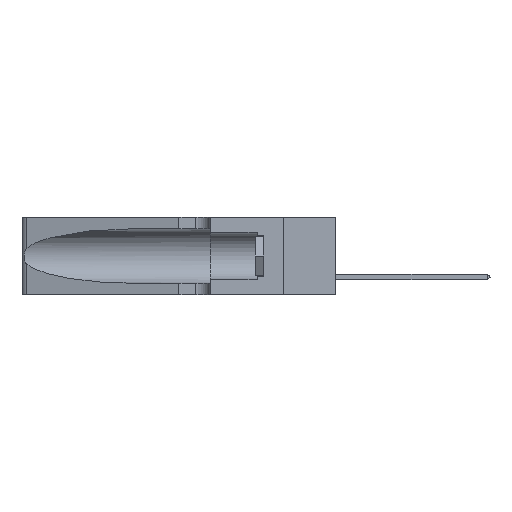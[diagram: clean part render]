
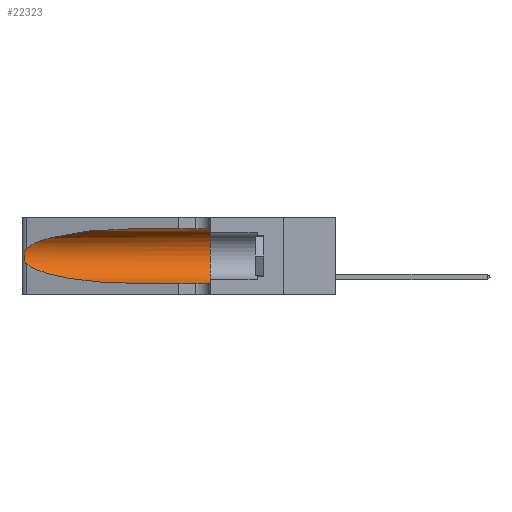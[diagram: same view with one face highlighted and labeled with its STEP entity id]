
A CAD part, left-side view. The second image highlights one B-rep face of the part: STEP entity #22323.
In plain terms, the highlighted cylindrical face has radius 3.308 mm (diameter 6.617 mm), a partial arc.
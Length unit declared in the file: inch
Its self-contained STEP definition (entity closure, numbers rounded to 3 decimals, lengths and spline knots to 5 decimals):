
#426 = ORIENTED_EDGE ( 'NONE', *, *, #15384, .F. ) ;
#1073 = DIRECTION ( 'NONE',  ( 0., 1., 0. ) ) ;
#1305 = CARTESIAN_POINT ( 'NONE',  ( 0.25487, 1.22718, 0.22369 ) ) ;
#1580 = VERTEX_POINT ( 'NONE', #9036 ) ;
#1773 = CARTESIAN_POINT ( 'NONE',  ( 0.18966, 0.96281, 0.05475 ) ) ;
#2220 =( BOUNDED_CURVE ( )  B_SPLINE_CURVE ( 3, ( #8843, #4147, #1773, #11015 ),
 .UNSPECIFIED., .F., .T. ) 
 B_SPLINE_CURVE_WITH_KNOTS ( ( 4, 4 ),
 ( 3.44316, 4.71239 ),
 .UNSPECIFIED. ) 
 CURVE ( )  GEOMETRIC_REPRESENTATION_ITEM ( )  RATIONAL_B_SPLINE_CURVE ( ( 1., 0.87, 0.87, 1. ) ) 
 REPRESENTATION_ITEM ( '' )  );
#3460 = CARTESIAN_POINT ( 'NONE',  ( 0.26075, 1.23896, 0.178 ) ) ;
#3535 = EDGE_CURVE ( 'NONE', #13968, #30046, #26366, .T. ) ;
#4147 = CARTESIAN_POINT ( 'NONE',  ( 0.2373, 1.15595, 0.08982 ) ) ;
#4462 = ORIENTED_EDGE ( 'NONE', *, *, #15866, .T. ) ;
#5500 = ORIENTED_EDGE ( 'NONE', *, *, #24151, .F. ) ;
#5898 = CARTESIAN_POINT ( 'NONE',  ( 0.25854, 1.2359, 0.20912 ) ) ;
#5960 = LINE ( 'NONE', #12563, #29646 ) ;
#5994 = EDGE_CURVE ( 'NONE', #21168, #13968, #2220, .T. ) ;
#6457 = B_SPLINE_CURVE_WITH_KNOTS ( 'NONE', 3,
 ( #1305, #10643, #25045, #27424, #5898, #15581, #17651, #3460, #22440, #8268, #13030, #17847, #24830, #22543 ),
 .UNSPECIFIED., .F., .F.,
 ( 4, 2, 2, 2, 2, 2, 4 ),
 ( 0., 0.00027, 0.00053, 0.00107, 0.0016, 0.00187, 0.00214 ),
 .UNSPECIFIED. ) ;
#7045 = FACE_OUTER_BOUND ( 'NONE', #24908, .T. ) ;
#8268 = CARTESIAN_POINT ( 'NONE',  ( 0.25856, 1.23593, 0.16098 ) ) ;
#8382 = ORIENTED_EDGE ( 'NONE', *, *, #21116, .T. ) ;
#8843 = CARTESIAN_POINT ( 'NONE',  ( 0.25487, 1.22718, 0.14631 ) ) ;
#9036 = CARTESIAN_POINT ( 'NONE',  ( 0.1305, 0.72297, 0.31525 ) ) ;
#9264 = ORIENTED_EDGE ( 'NONE', *, *, #5994, .T. ) ;
#10340 = CARTESIAN_POINT ( 'NONE',  ( 0.1305, 1.61858, 0.185 ) ) ;
#10548 = DIRECTION ( 'NONE',  ( 0., 0., -1. ) ) ;
#10643 = CARTESIAN_POINT ( 'NONE',  ( 0.25555, 1.22994, 0.2215 ) ) ;
#10761 = DIRECTION ( 'NONE',  ( 0., -1., 0. ) ) ;
#10962 = CARTESIAN_POINT ( 'NONE',  ( 0.25487, 1.22718, 0.14631 ) ) ;
#11015 = CARTESIAN_POINT ( 'NONE',  ( 0.1305, 0.72297, 0.05475 ) ) ;
#12563 = CARTESIAN_POINT ( 'NONE',  ( 0.1305, 1.61858, 0.31525 ) ) ;
#13030 = CARTESIAN_POINT ( 'NONE',  ( 0.25789, 1.23486, 0.15765 ) ) ;
#13726 = CARTESIAN_POINT ( 'NONE',  ( 0.18966, 0.96281, 0.31525 ) ) ;
#13968 = VERTEX_POINT ( 'NONE', #14469 ) ;
#14469 = CARTESIAN_POINT ( 'NONE',  ( 0.1305, 0.72297, 0.05475 ) ) ;
#14495 = VECTOR ( 'NONE', #24199, 39.37008 ) ;
#14793 = CYLINDRICAL_SURFACE ( 'NONE', #16896, 0.13025 ) ;
#15261 = CARTESIAN_POINT ( 'NONE',  ( 0.1305, 0.35, 0.185 ) ) ;
#15384 = EDGE_CURVE ( 'NONE', #1580, #29355, #5960, .T. ) ;
#15581 = CARTESIAN_POINT ( 'NONE',  ( 0.26018, 1.23835, 0.19895 ) ) ;
#15806 = AXIS2_PLACEMENT_3D ( 'NONE', #15261, #1073, #19334 ) ;
#15866 = EDGE_CURVE ( 'NONE', #1580, #20215, #21050, .T. ) ;
#16100 = CARTESIAN_POINT ( 'NONE',  ( 0.2373, 1.15595, 0.28018 ) ) ;
#16394 = CARTESIAN_POINT ( 'NONE',  ( 0.1305, 0.72297, 0.31525 ) ) ;
#16896 = AXIS2_PLACEMENT_3D ( 'NONE', #10340, #10761, #10548 ) ;
#17651 = CARTESIAN_POINT ( 'NONE',  ( 0.26075, 1.23896, 0.19203 ) ) ;
#17847 = CARTESIAN_POINT ( 'NONE',  ( 0.25639, 1.23186, 0.15144 ) ) ;
#18046 = ORIENTED_EDGE ( 'NONE', *, *, #3535, .T. ) ;
#18467 = CARTESIAN_POINT ( 'NONE',  ( 0.25487, 1.22718, 0.22369 ) ) ;
#19334 = DIRECTION ( 'NONE',  ( 0., 0., 1. ) ) ;
#19395 = CARTESIAN_POINT ( 'NONE',  ( 0.1305, 1.61858, 0.05475 ) ) ;
#19982 = DIRECTION ( 'NONE',  ( 0., -1., 0. ) ) ;
#20215 = VERTEX_POINT ( 'NONE', #18467 ) ;
#20618 = CIRCLE ( 'NONE', #15806, 0.13025 ) ;
#20868 = CARTESIAN_POINT ( 'NONE',  ( 0.25487, 1.22718, 0.22369 ) ) ;
#21050 =( BOUNDED_CURVE ( )  B_SPLINE_CURVE ( 3, ( #16394, #13726, #16100, #20868 ),
 .UNSPECIFIED., .F., .F. ) 
 B_SPLINE_CURVE_WITH_KNOTS ( ( 4, 4 ),
 ( 1.5708, 2.84003 ),
 .UNSPECIFIED. ) 
 CURVE ( )  GEOMETRIC_REPRESENTATION_ITEM ( )  RATIONAL_B_SPLINE_CURVE ( ( 1., 0.87, 0.87, 1. ) ) 
 REPRESENTATION_ITEM ( '' )  );
#21116 = EDGE_CURVE ( 'NONE', #20215, #21168, #6457, .T. ) ;
#21168 = VERTEX_POINT ( 'NONE', #10962 ) ;
#22323 = ADVANCED_FACE ( 'NONE', ( #7045 ), #14793, .F. ) ;
#22440 = CARTESIAN_POINT ( 'NONE',  ( 0.26017, 1.23833, 0.17102 ) ) ;
#22543 = CARTESIAN_POINT ( 'NONE',  ( 0.25487, 1.22718, 0.14631 ) ) ;
#24151 = EDGE_CURVE ( 'NONE', #29355, #30046, #20618, .T. ) ;
#24199 = DIRECTION ( 'NONE',  ( 0., -1., 0. ) ) ;
#24830 = CARTESIAN_POINT ( 'NONE',  ( 0.25555, 1.22993, 0.14849 ) ) ;
#24908 = EDGE_LOOP ( 'NONE', ( #4462, #8382, #9264, #18046, #5500, #426 ) ) ;
#25045 = CARTESIAN_POINT ( 'NONE',  ( 0.25639, 1.23184, 0.21858 ) ) ;
#26366 = LINE ( 'NONE', #19395, #14495 ) ;
#27424 = CARTESIAN_POINT ( 'NONE',  ( 0.25787, 1.23484, 0.2124 ) ) ;
#28901 = CARTESIAN_POINT ( 'NONE',  ( 0.1305, 0.35, 0.31525 ) ) ;
#29297 = CARTESIAN_POINT ( 'NONE',  ( 0.1305, 0.35, 0.05475 ) ) ;
#29355 = VERTEX_POINT ( 'NONE', #28901 ) ;
#29646 = VECTOR ( 'NONE', #19982, 39.37008 ) ;
#30046 = VERTEX_POINT ( 'NONE', #29297 ) ;
